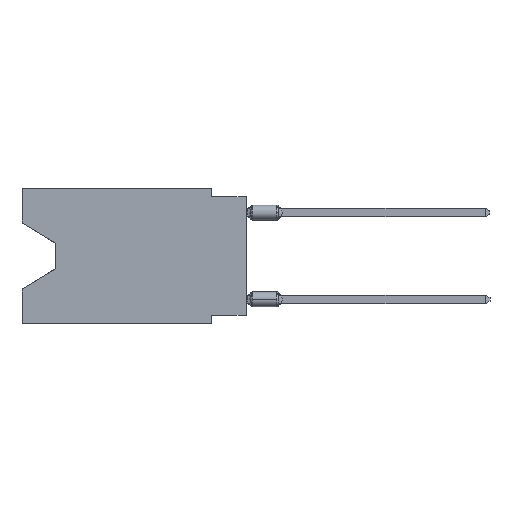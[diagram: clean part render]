
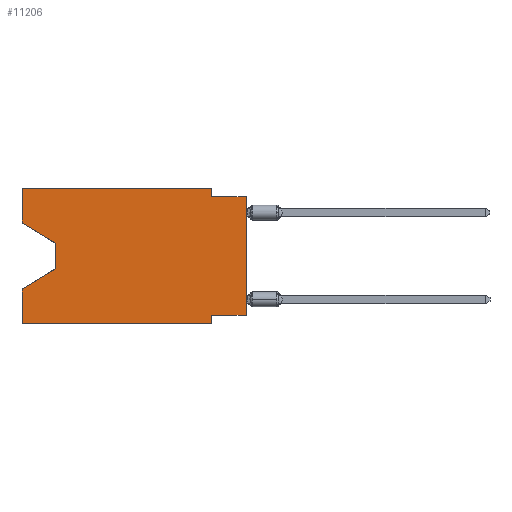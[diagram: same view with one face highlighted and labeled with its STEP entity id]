
A CAD part, left-side view. The second image highlights one B-rep face of the part: STEP entity #11206.
In plain terms, the highlighted planar face has unit normal (-1, 0, 0).
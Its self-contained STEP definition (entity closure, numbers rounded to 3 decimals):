
#58 = CARTESIAN_POINT ( 'NONE',  ( 0., 16.383, -2.546 ) ) ;
#90 = LINE ( 'NONE', #13239, #10955 ) ;
#189 = ORIENTED_EDGE ( 'NONE', *, *, #9819, .T. ) ;
#569 = EDGE_CURVE ( 'NONE', #4877, #4488, #1300, .T. ) ;
#898 = CARTESIAN_POINT ( 'NONE',  ( 0., 13.97, -4.013 ) ) ;
#936 = ORIENTED_EDGE ( 'NONE', *, *, #569, .F. ) ;
#1131 = CARTESIAN_POINT ( 'NONE',  ( 0., 16.383, 0. ) ) ;
#1300 = LINE ( 'NONE', #5125, #2412 ) ;
#1512 = CARTESIAN_POINT ( 'NONE',  ( 0., 16.383, -9.906 ) ) ;
#1551 = VERTEX_POINT ( 'NONE', #10708 ) ;
#1558 = DIRECTION ( 'NONE',  ( 0., 0., -1. ) ) ;
#1634 = ORIENTED_EDGE ( 'NONE', *, *, #9831, .T. ) ;
#1955 = ORIENTED_EDGE ( 'NONE', *, *, #2213, .F. ) ;
#2213 = EDGE_CURVE ( 'NONE', #17072, #4877, #13200, .T. ) ;
#2412 = VECTOR ( 'NONE', #4882, 1000. ) ;
#2477 = VERTEX_POINT ( 'NONE', #898 ) ;
#2790 = CARTESIAN_POINT ( 'NONE',  ( 0., 13.97, -5.893 ) ) ;
#2904 = VECTOR ( 'NONE', #12819, 1000. ) ;
#2974 = DIRECTION ( 'NONE',  ( 0., 0.855, -0.519 ) ) ;
#3203 = AXIS2_PLACEMENT_3D ( 'NONE', #1131, #7578, #10443 ) ;
#3279 = CARTESIAN_POINT ( 'NONE',  ( 0., 13.97, -5.893 ) ) ;
#3340 = CARTESIAN_POINT ( 'NONE',  ( 0., 0., 0. ) ) ;
#3611 = LINE ( 'NONE', #6209, #11865 ) ;
#3930 = VECTOR ( 'NONE', #16054, 1000. ) ;
#3953 = ORIENTED_EDGE ( 'NONE', *, *, #7068, .F. ) ;
#4263 = VECTOR ( 'NONE', #2974, 1000. ) ;
#4282 = ORIENTED_EDGE ( 'NONE', *, *, #5149, .T. ) ;
#4465 = LINE ( 'NONE', #3340, #2904 ) ;
#4488 = VERTEX_POINT ( 'NONE', #5909 ) ;
#4877 = VERTEX_POINT ( 'NONE', #8866 ) ;
#4882 = DIRECTION ( 'NONE',  ( 0., -1., 0. ) ) ;
#5125 = CARTESIAN_POINT ( 'NONE',  ( 0., 0., -0.635 ) ) ;
#5149 = EDGE_CURVE ( 'NONE', #7866, #4488, #4465, .T. ) ;
#5648 = DIRECTION ( 'NONE',  ( 0., -0.855, -0.519 ) ) ;
#5851 = DIRECTION ( 'NONE',  ( 0., -1., 0. ) ) ;
#5909 = CARTESIAN_POINT ( 'NONE',  ( 0., 0., -0.635 ) ) ;
#6209 = CARTESIAN_POINT ( 'NONE',  ( 0., 16.383, 0. ) ) ;
#6366 = FACE_OUTER_BOUND ( 'NONE', #15323, .T. ) ;
#6486 = DIRECTION ( 'NONE',  ( 0., 0., -1. ) ) ;
#6671 = VERTEX_POINT ( 'NONE', #58 ) ;
#6865 = EDGE_CURVE ( 'NONE', #7866, #13280, #9774, .T. ) ;
#6892 = LINE ( 'NONE', #9489, #10660 ) ;
#6896 = VECTOR ( 'NONE', #6486, 1000. ) ;
#7068 = EDGE_CURVE ( 'NONE', #13514, #15088, #3611, .T. ) ;
#7284 = VECTOR ( 'NONE', #8733, 1000. ) ;
#7578 = DIRECTION ( 'NONE',  ( 1., 0., 0. ) ) ;
#7833 = CARTESIAN_POINT ( 'NONE',  ( 0., 16.383, -9.906 ) ) ;
#7866 = VERTEX_POINT ( 'NONE', #8765 ) ;
#8682 = ORIENTED_EDGE ( 'NONE', *, *, #12492, .T. ) ;
#8695 = CARTESIAN_POINT ( 'NONE',  ( 0., 16.383, 0. ) ) ;
#8733 = DIRECTION ( 'NONE',  ( 0., 0., 1. ) ) ;
#8765 = CARTESIAN_POINT ( 'NONE',  ( 0., 0., -9.271 ) ) ;
#8866 = CARTESIAN_POINT ( 'NONE',  ( 0., 2.54, -0.635 ) ) ;
#9226 = DIRECTION ( 'NONE',  ( 0., -1., 0. ) ) ;
#9416 = LINE ( 'NONE', #2790, #4263 ) ;
#9489 = CARTESIAN_POINT ( 'NONE',  ( 0., 16.383, -2.546 ) ) ;
#9774 = LINE ( 'NONE', #11178, #10999 ) ;
#9819 = EDGE_CURVE ( 'NONE', #6671, #2477, #6892, .T. ) ;
#9831 = EDGE_CURVE ( 'NONE', #16633, #15088, #9416, .T. ) ;
#9874 = DIRECTION ( 'NONE',  ( 0., 1., 0. ) ) ;
#10277 = EDGE_CURVE ( 'NONE', #2477, #16633, #90, .T. ) ;
#10443 = DIRECTION ( 'NONE',  ( 0., 0., -1. ) ) ;
#10660 = VECTOR ( 'NONE', #5648, 1000. ) ;
#10708 = CARTESIAN_POINT ( 'NONE',  ( 0., 2.54, -9.906 ) ) ;
#10837 = LINE ( 'NONE', #14591, #3930 ) ;
#10955 = VECTOR ( 'NONE', #1558, 1000. ) ;
#10999 = VECTOR ( 'NONE', #9874, 1000. ) ;
#11088 = LINE ( 'NONE', #12549, #11716 ) ;
#11178 = CARTESIAN_POINT ( 'NONE',  ( 0., 0., -9.271 ) ) ;
#11205 = ORIENTED_EDGE ( 'NONE', *, *, #6865, .F. ) ;
#11206 = ADVANCED_FACE ( 'NONE', ( #6366 ), #15499, .F. ) ;
#11716 = VECTOR ( 'NONE', #5851, 1000. ) ;
#11865 = VECTOR ( 'NONE', #15848, 1000. ) ;
#12097 = ORIENTED_EDGE ( 'NONE', *, *, #14791, .F. ) ;
#12109 = EDGE_CURVE ( 'NONE', #13280, #1551, #10837, .T. ) ;
#12199 = EDGE_CURVE ( 'NONE', #15550, #17072, #11088, .T. ) ;
#12492 = EDGE_CURVE ( 'NONE', #13514, #1551, #14541, .T. ) ;
#12549 = CARTESIAN_POINT ( 'NONE',  ( 0., 16.383, 0. ) ) ;
#12819 = DIRECTION ( 'NONE',  ( 0., 0., 1. ) ) ;
#13097 = ORIENTED_EDGE ( 'NONE', *, *, #10277, .T. ) ;
#13200 = LINE ( 'NONE', #14334, #6896 ) ;
#13239 = CARTESIAN_POINT ( 'NONE',  ( 0., 13.97, -4.013 ) ) ;
#13280 = VERTEX_POINT ( 'NONE', #13899 ) ;
#13514 = VERTEX_POINT ( 'NONE', #1512 ) ;
#13899 = CARTESIAN_POINT ( 'NONE',  ( 0., 2.54, -9.271 ) ) ;
#14144 = LINE ( 'NONE', #16475, #7284 ) ;
#14334 = CARTESIAN_POINT ( 'NONE',  ( 0., 2.54, 0. ) ) ;
#14541 = LINE ( 'NONE', #7833, #16438 ) ;
#14591 = CARTESIAN_POINT ( 'NONE',  ( 0., 2.54, -9.906 ) ) ;
#14791 = EDGE_CURVE ( 'NONE', #6671, #15550, #14144, .T. ) ;
#15088 = VERTEX_POINT ( 'NONE', #15947 ) ;
#15162 = ORIENTED_EDGE ( 'NONE', *, *, #12199, .F. ) ;
#15323 = EDGE_LOOP ( 'NONE', ( #189, #13097, #1634, #3953, #8682, #15411, #11205, #4282, #936, #1955, #15162, #12097 ) ) ;
#15411 = ORIENTED_EDGE ( 'NONE', *, *, #12109, .F. ) ;
#15499 = PLANE ( 'NONE',  #3203 ) ;
#15550 = VERTEX_POINT ( 'NONE', #8695 ) ;
#15848 = DIRECTION ( 'NONE',  ( 0., 0., 1. ) ) ;
#15947 = CARTESIAN_POINT ( 'NONE',  ( 0., 16.383, -7.36 ) ) ;
#16054 = DIRECTION ( 'NONE',  ( 0., 0., -1. ) ) ;
#16438 = VECTOR ( 'NONE', #9226, 1000. ) ;
#16475 = CARTESIAN_POINT ( 'NONE',  ( 0., 16.383, 0. ) ) ;
#16633 = VERTEX_POINT ( 'NONE', #3279 ) ;
#16892 = CARTESIAN_POINT ( 'NONE',  ( 0., 2.54, 0. ) ) ;
#17072 = VERTEX_POINT ( 'NONE', #16892 ) ;
